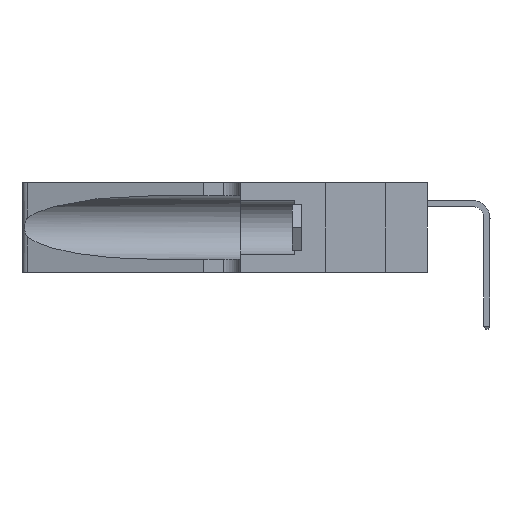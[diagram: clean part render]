
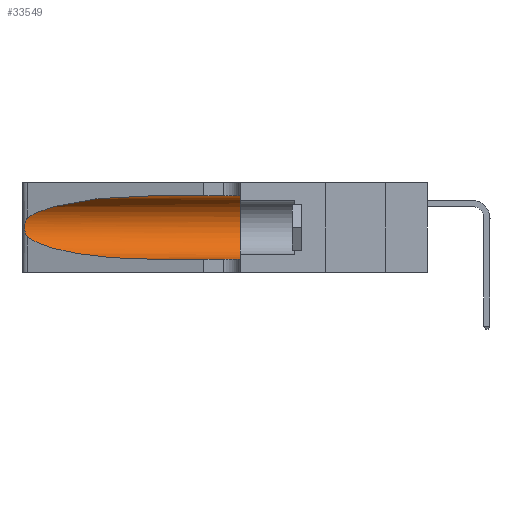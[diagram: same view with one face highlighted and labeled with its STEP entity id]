
A CAD part, left-side view. The second image highlights one B-rep face of the part: STEP entity #33549.
In plain terms, the highlighted cylindrical face has radius 3.308 mm (diameter 6.617 mm), a partial arc.
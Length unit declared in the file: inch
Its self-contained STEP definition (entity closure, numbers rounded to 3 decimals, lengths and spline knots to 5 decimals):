
#63 = CARTESIAN_POINT ( 'NONE',  ( 0.25487, 1.22718, 0.22369 ) ) ;
#184 = CARTESIAN_POINT ( 'NONE',  ( 0.25856, 1.23593, 0.16098 ) ) ;
#462 = AXIS2_PLACEMENT_3D ( 'NONE', #38029, #5106, #26242 ) ;
#570 = AXIS2_PLACEMENT_3D ( 'NONE', #24391, #6317, #27452 ) ;
#920 = B_SPLINE_CURVE_WITH_KNOTS ( 'NONE', 3,
 ( #63, #21179, #9159, #30300, #12161, #33271, #15195, #36239, #18268, #184, #21310, #3274, #24349, #6279 ),
 .UNSPECIFIED., .F., .F.,
 ( 4, 2, 2, 2, 2, 2, 4 ),
 ( 0., 0.00027, 0.00053, 0.00107, 0.0016, 0.00187, 0.00214 ),
 .UNSPECIFIED. ) ;
#1451 = EDGE_CURVE ( 'NONE', #4353, #1782, #1593, .T. ) ;
#1558 = CARTESIAN_POINT ( 'NONE',  ( 0.1305, 0.35, 0.31525 ) ) ;
#1593 = LINE ( 'NONE', #24780, #18559 ) ;
#1782 = VERTEX_POINT ( 'NONE', #32232 ) ;
#3233 = EDGE_CURVE ( 'NONE', #30244, #1782, #33490, .T. ) ;
#3274 = CARTESIAN_POINT ( 'NONE',  ( 0.25639, 1.23186, 0.15144 ) ) ;
#3538 = CARTESIAN_POINT ( 'NONE',  ( 0.1305, 0.72297, 0.31525 ) ) ;
#3702 = DIRECTION ( 'NONE',  ( 0., -1., 0. ) ) ;
#4353 = VERTEX_POINT ( 'NONE', #28163 ) ;
#4593 = VERTEX_POINT ( 'NONE', #8049 ) ;
#5106 = DIRECTION ( 'NONE',  ( 0., -1., 0. ) ) ;
#6279 = CARTESIAN_POINT ( 'NONE',  ( 0.25487, 1.22718, 0.14631 ) ) ;
#6317 = DIRECTION ( 'NONE',  ( 0., 1., 0. ) ) ;
#6544 = CARTESIAN_POINT ( 'NONE',  ( 0.2373, 1.15595, 0.28018 ) ) ;
#6579 = CARTESIAN_POINT ( 'NONE',  ( 0.1305, 1.61858, 0.31525 ) ) ;
#6963 = CARTESIAN_POINT ( 'NONE',  ( 0.18966, 0.96281, 0.05475 ) ) ;
#8049 = CARTESIAN_POINT ( 'NONE',  ( 0.1305, 0.72297, 0.31525 ) ) ;
#8182 =( BOUNDED_CURVE ( )  B_SPLINE_CURVE ( 3, ( #30980, #22014, #6963, #28114 ),
 .UNSPECIFIED., .F., .T. ) 
 B_SPLINE_CURVE_WITH_KNOTS ( ( 4, 4 ),
 ( 3.44316, 4.71239 ),
 .UNSPECIFIED. ) 
 CURVE ( )  GEOMETRIC_REPRESENTATION_ITEM ( )  RATIONAL_B_SPLINE_CURVE ( ( 1., 0.87, 0.87, 1. ) ) 
 REPRESENTATION_ITEM ( '' )  );
#9159 = CARTESIAN_POINT ( 'NONE',  ( 0.25639, 1.23184, 0.21858 ) ) ;
#9390 =( BOUNDED_CURVE ( )  B_SPLINE_CURVE ( 3, ( #3538, #12425, #6544, #27677 ),
 .UNSPECIFIED., .F., .T. ) 
 B_SPLINE_CURVE_WITH_KNOTS ( ( 4, 4 ),
 ( 1.5708, 2.84003 ),
 .UNSPECIFIED. ) 
 CURVE ( )  GEOMETRIC_REPRESENTATION_ITEM ( )  RATIONAL_B_SPLINE_CURVE ( ( 1., 0.87, 0.87, 1. ) ) 
 REPRESENTATION_ITEM ( '' )  );
#11901 = EDGE_CURVE ( 'NONE', #4593, #38298, #9390, .T. ) ;
#12161 = CARTESIAN_POINT ( 'NONE',  ( 0.25854, 1.2359, 0.20912 ) ) ;
#12425 = CARTESIAN_POINT ( 'NONE',  ( 0.18966, 0.96281, 0.31525 ) ) ;
#12579 = EDGE_CURVE ( 'NONE', #34926, #4353, #8182, .T. ) ;
#14453 = CARTESIAN_POINT ( 'NONE',  ( 0.25487, 1.22718, 0.14631 ) ) ;
#15195 = CARTESIAN_POINT ( 'NONE',  ( 0.26075, 1.23896, 0.19203 ) ) ;
#17094 = FACE_OUTER_BOUND ( 'NONE', #19587, .T. ) ;
#17219 = CARTESIAN_POINT ( 'NONE',  ( 0.25487, 1.22718, 0.22369 ) ) ;
#17883 = VECTOR ( 'NONE', #24795, 39.37008 ) ;
#18126 = ORIENTED_EDGE ( 'NONE', *, *, #1451, .T. ) ;
#18268 = CARTESIAN_POINT ( 'NONE',  ( 0.26017, 1.23833, 0.17102 ) ) ;
#18559 = VECTOR ( 'NONE', #3702, 39.37008 ) ;
#19394 = ORIENTED_EDGE ( 'NONE', *, *, #30044, .F. ) ;
#19587 = EDGE_LOOP ( 'NONE', ( #36217, #30692, #30864, #18126, #28585, #19394 ) ) ;
#21179 = CARTESIAN_POINT ( 'NONE',  ( 0.25555, 1.22994, 0.2215 ) ) ;
#21310 = CARTESIAN_POINT ( 'NONE',  ( 0.25789, 1.23486, 0.15765 ) ) ;
#22014 = CARTESIAN_POINT ( 'NONE',  ( 0.2373, 1.15595, 0.08982 ) ) ;
#23240 = CYLINDRICAL_SURFACE ( 'NONE', #462, 0.13025 ) ;
#24349 = CARTESIAN_POINT ( 'NONE',  ( 0.25555, 1.22993, 0.14849 ) ) ;
#24391 = CARTESIAN_POINT ( 'NONE',  ( 0.1305, 0.35, 0.185 ) ) ;
#24745 = EDGE_CURVE ( 'NONE', #38298, #34926, #920, .T. ) ;
#24780 = CARTESIAN_POINT ( 'NONE',  ( 0.1305, 1.61858, 0.05475 ) ) ;
#24795 = DIRECTION ( 'NONE',  ( 0., -1., 0. ) ) ;
#26242 = DIRECTION ( 'NONE',  ( 0., 0., -1. ) ) ;
#27452 = DIRECTION ( 'NONE',  ( 0., 0., 1. ) ) ;
#27677 = CARTESIAN_POINT ( 'NONE',  ( 0.25487, 1.22718, 0.22369 ) ) ;
#28114 = CARTESIAN_POINT ( 'NONE',  ( 0.1305, 0.72297, 0.05475 ) ) ;
#28163 = CARTESIAN_POINT ( 'NONE',  ( 0.1305, 0.72297, 0.05475 ) ) ;
#28585 = ORIENTED_EDGE ( 'NONE', *, *, #3233, .F. ) ;
#30044 = EDGE_CURVE ( 'NONE', #4593, #30244, #33892, .T. ) ;
#30244 = VERTEX_POINT ( 'NONE', #1558 ) ;
#30300 = CARTESIAN_POINT ( 'NONE',  ( 0.25787, 1.23484, 0.2124 ) ) ;
#30692 = ORIENTED_EDGE ( 'NONE', *, *, #24745, .T. ) ;
#30864 = ORIENTED_EDGE ( 'NONE', *, *, #12579, .T. ) ;
#30980 = CARTESIAN_POINT ( 'NONE',  ( 0.25487, 1.22718, 0.14631 ) ) ;
#32232 = CARTESIAN_POINT ( 'NONE',  ( 0.1305, 0.35, 0.05475 ) ) ;
#33271 = CARTESIAN_POINT ( 'NONE',  ( 0.26018, 1.23835, 0.19895 ) ) ;
#33490 = CIRCLE ( 'NONE', #570, 0.13025 ) ;
#33549 = ADVANCED_FACE ( 'NONE', ( #17094 ), #23240, .F. ) ;
#33892 = LINE ( 'NONE', #6579, #17883 ) ;
#34926 = VERTEX_POINT ( 'NONE', #14453 ) ;
#36217 = ORIENTED_EDGE ( 'NONE', *, *, #11901, .T. ) ;
#36239 = CARTESIAN_POINT ( 'NONE',  ( 0.26075, 1.23896, 0.178 ) ) ;
#38029 = CARTESIAN_POINT ( 'NONE',  ( 0.1305, 1.61858, 0.185 ) ) ;
#38298 = VERTEX_POINT ( 'NONE', #17219 ) ;
